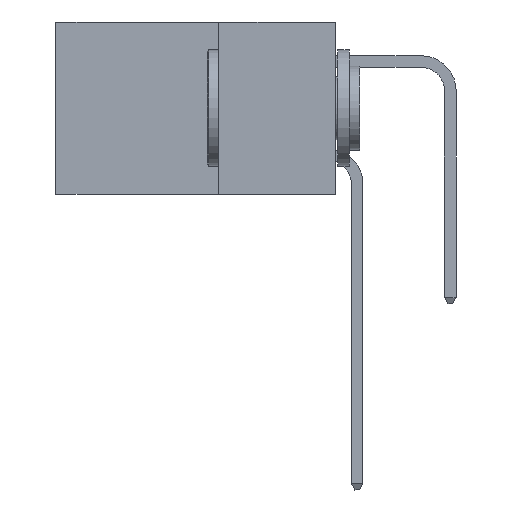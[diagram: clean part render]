
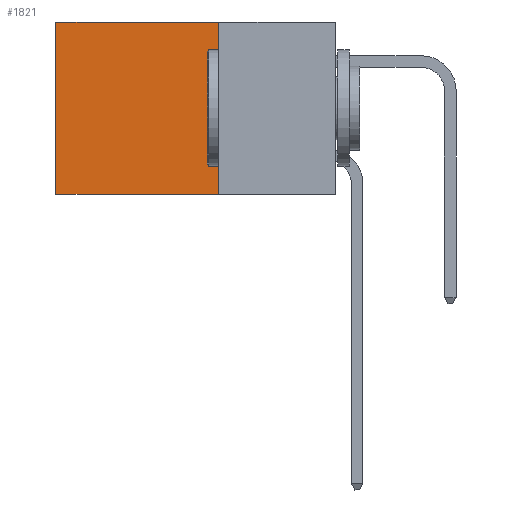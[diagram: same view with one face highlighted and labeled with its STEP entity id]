
A CAD part, left-side view. The second image highlights one B-rep face of the part: STEP entity #1821.
In plain terms, the highlighted planar face has unit normal (-1, 0, 0).
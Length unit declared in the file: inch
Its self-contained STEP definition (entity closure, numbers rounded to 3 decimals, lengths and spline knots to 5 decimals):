
#130 = PLANE ( 'NONE',  #1511 ) ;
#493 = VECTOR ( 'NONE', #3803, 39.37008 ) ;
#1119 = LINE ( 'NONE', #6791, #493 ) ;
#1178 = DIRECTION ( 'NONE',  ( 0., 0., -1. ) ) ;
#1511 = AXIS2_PLACEMENT_3D ( 'NONE', #7504, #4933, #1178 ) ;
#1821 = ADVANCED_FACE ( 'NONE', ( #8106 ), #130, .F. ) ;
#1877 = LINE ( 'NONE', #8353, #3679 ) ;
#2251 = CARTESIAN_POINT ( 'NONE',  ( 0.2875, 0.25, -0.37 ) ) ;
#2920 = VERTEX_POINT ( 'NONE', #4649 ) ;
#3679 = VECTOR ( 'NONE', #6624, 39.37008 ) ;
#3772 = VERTEX_POINT ( 'NONE', #12263 ) ;
#3803 = DIRECTION ( 'NONE',  ( 0., 1., 0. ) ) ;
#3893 = EDGE_CURVE ( 'NONE', #3772, #7832, #1877, .T. ) ;
#4309 = VECTOR ( 'NONE', #6104, 39.37008 ) ;
#4649 = CARTESIAN_POINT ( 'NONE',  ( 0.2875, 0.6, 0. ) ) ;
#4792 = VERTEX_POINT ( 'NONE', #11438 ) ;
#4933 = DIRECTION ( 'NONE',  ( 1., 0., 0. ) ) ;
#6104 = DIRECTION ( 'NONE',  ( 0., 1., 0. ) ) ;
#6383 = ORIENTED_EDGE ( 'NONE', *, *, #12208, .F. ) ;
#6624 = DIRECTION ( 'NONE',  ( 0., 0., -1. ) ) ;
#6740 = LINE ( 'NONE', #10106, #12359 ) ;
#6791 = CARTESIAN_POINT ( 'NONE',  ( 0.2875, 0.25, 0. ) ) ;
#7504 = CARTESIAN_POINT ( 'NONE',  ( 0.2875, 0.25, 0. ) ) ;
#7832 = VERTEX_POINT ( 'NONE', #2251 ) ;
#8026 = ORIENTED_EDGE ( 'NONE', *, *, #10668, .T. ) ;
#8106 = FACE_OUTER_BOUND ( 'NONE', #11811, .T. ) ;
#8144 = ORIENTED_EDGE ( 'NONE', *, *, #8588, .T. ) ;
#8353 = CARTESIAN_POINT ( 'NONE',  ( 0.2875, 0.25, 0. ) ) ;
#8588 = EDGE_CURVE ( 'NONE', #2920, #4792, #6740, .T. ) ;
#9806 = ORIENTED_EDGE ( 'NONE', *, *, #3893, .F. ) ;
#9913 = CARTESIAN_POINT ( 'NONE',  ( 0.2875, 0.25, -0.37 ) ) ;
#10106 = CARTESIAN_POINT ( 'NONE',  ( 0.2875, 0.6, 0. ) ) ;
#10668 = EDGE_CURVE ( 'NONE', #3772, #2920, #1119, .T. ) ;
#11081 = DIRECTION ( 'NONE',  ( 0., 0., -1. ) ) ;
#11438 = CARTESIAN_POINT ( 'NONE',  ( 0.2875, 0.6, -0.37 ) ) ;
#11746 = LINE ( 'NONE', #9913, #4309 ) ;
#11811 = EDGE_LOOP ( 'NONE', ( #8144, #6383, #9806, #8026 ) ) ;
#12208 = EDGE_CURVE ( 'NONE', #7832, #4792, #11746, .T. ) ;
#12263 = CARTESIAN_POINT ( 'NONE',  ( 0.2875, 0.25, 0. ) ) ;
#12359 = VECTOR ( 'NONE', #11081, 39.37008 ) ;
